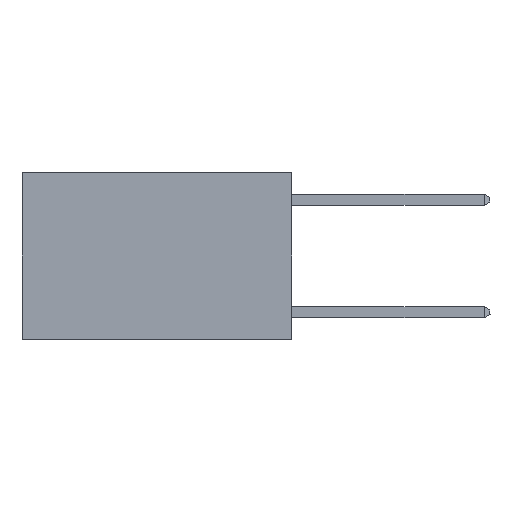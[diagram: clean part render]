
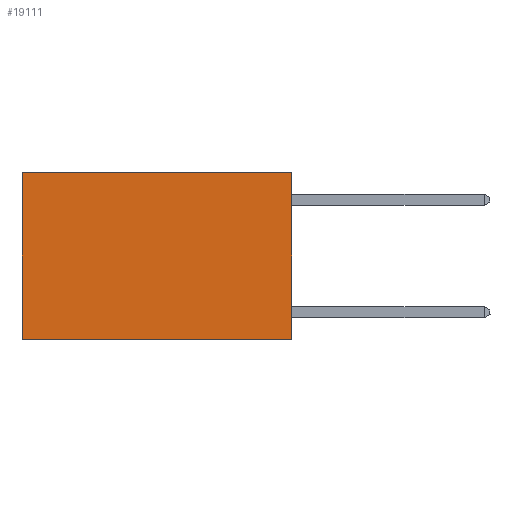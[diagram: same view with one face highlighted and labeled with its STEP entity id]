
A CAD part, left-side view. The second image highlights one B-rep face of the part: STEP entity #19111.
In plain terms, the highlighted planar face has unit normal (-1, 0, 0).
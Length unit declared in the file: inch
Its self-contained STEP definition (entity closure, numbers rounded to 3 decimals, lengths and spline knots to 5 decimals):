
#269 = CARTESIAN_POINT ( 'NONE',  ( 0.2625, 0., -0.37 ) ) ;
#862 = EDGE_CURVE ( 'NONE', #1134, #18648, #18937, .T. ) ;
#1134 = VERTEX_POINT ( 'NONE', #11452 ) ;
#1147 = CARTESIAN_POINT ( 'NONE',  ( 0.2625, 0.6, 0. ) ) ;
#4000 = ORIENTED_EDGE ( 'NONE', *, *, #862, .T. ) ;
#4518 = LINE ( 'NONE', #10771, #8232 ) ;
#5027 = ORIENTED_EDGE ( 'NONE', *, *, #11534, .T. ) ;
#5029 = DIRECTION ( 'NONE',  ( 0., 0., -1. ) ) ;
#5691 = LINE ( 'NONE', #13641, #6721 ) ;
#6721 = VECTOR ( 'NONE', #21548, 39.37008 ) ;
#6935 = CARTESIAN_POINT ( 'NONE',  ( 0.2625, 0., 0. ) ) ;
#7414 = CARTESIAN_POINT ( 'NONE',  ( 0.2625, 0.6, -0.37 ) ) ;
#8232 = VECTOR ( 'NONE', #14937, 39.37008 ) ;
#9139 = LINE ( 'NONE', #17055, #12187 ) ;
#10771 = CARTESIAN_POINT ( 'NONE',  ( 0.2625, 0., 0. ) ) ;
#10787 = EDGE_CURVE ( 'NONE', #22055, #18648, #5691, .T. ) ;
#11452 = CARTESIAN_POINT ( 'NONE',  ( 0.2625, 0.6, 0. ) ) ;
#11534 = EDGE_CURVE ( 'NONE', #17988, #1134, #9139, .T. ) ;
#12187 = VECTOR ( 'NONE', #21076, 39.37008 ) ;
#13641 = CARTESIAN_POINT ( 'NONE',  ( 0.2625, 0., -0.37 ) ) ;
#14937 = DIRECTION ( 'NONE',  ( 0., 0., -1. ) ) ;
#15316 = VECTOR ( 'NONE', #5029, 39.37008 ) ;
#15462 = DIRECTION ( 'NONE',  ( 1., 0., 0. ) ) ;
#17055 = CARTESIAN_POINT ( 'NONE',  ( 0.2625, 0., 0. ) ) ;
#17225 = ORIENTED_EDGE ( 'NONE', *, *, #10787, .F. ) ;
#17395 = FACE_OUTER_BOUND ( 'NONE', #17938, .T. ) ;
#17938 = EDGE_LOOP ( 'NONE', ( #4000, #17225, #23444, #5027 ) ) ;
#17988 = VERTEX_POINT ( 'NONE', #6935 ) ;
#18648 = VERTEX_POINT ( 'NONE', #7414 ) ;
#18937 = LINE ( 'NONE', #1147, #15316 ) ;
#19111 = ADVANCED_FACE ( 'NONE', ( #17395 ), #19589, .F. ) ;
#19589 = PLANE ( 'NONE',  #23428 ) ;
#21076 = DIRECTION ( 'NONE',  ( 0., 1., 0. ) ) ;
#21423 = CARTESIAN_POINT ( 'NONE',  ( 0.2625, 0., 0. ) ) ;
#21548 = DIRECTION ( 'NONE',  ( 0., 1., 0. ) ) ;
#22055 = VERTEX_POINT ( 'NONE', #269 ) ;
#23375 = DIRECTION ( 'NONE',  ( 0., 0., -1. ) ) ;
#23428 = AXIS2_PLACEMENT_3D ( 'NONE', #21423, #15462, #23375 ) ;
#23444 = ORIENTED_EDGE ( 'NONE', *, *, #25516, .F. ) ;
#25516 = EDGE_CURVE ( 'NONE', #17988, #22055, #4518, .T. ) ;
